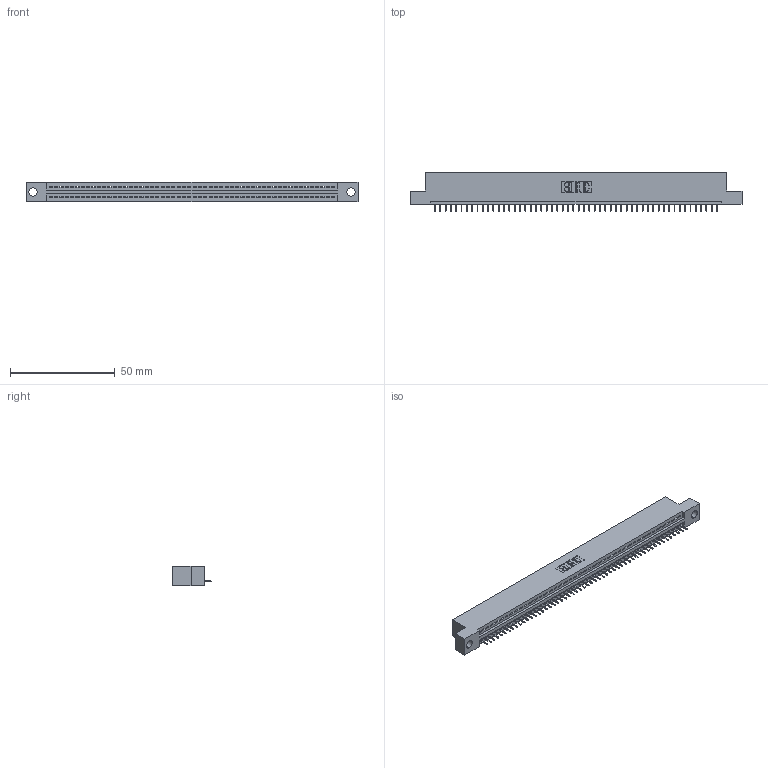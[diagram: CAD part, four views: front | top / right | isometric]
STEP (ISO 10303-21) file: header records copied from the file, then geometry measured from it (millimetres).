
FILE_DESCRIPTION (( 'STEP AP203' ), '1' );
FILE_NAME ('895-054-525-104.STEP', '2020-09-27T13:54:19', ( '' ), ( '' ), 'SwSTEP 2.0', 'SolidWorks 2020', '' );
FILE_SCHEMA (( 'CONFIG_CONTROL_DESIGN' ));
Length unit declared in the file: inch
Products named in the file (3): 345-292-001_345-293-125; 845 Part_Flush Mounting Lugs - 0.156 Dia-TH; 895-054-525-104
Assembly tree (55 placements, depth 2):
  895-054-525-104
    845 Part_Flush Mounting Lugs - 0.156 Dia-TH
    345-292-001_345-293-125  x54
Bounding box: 158.37 x 18.72 x 9.4 mm (x, y, z)
Volume: 14832 mm3; surface area: 18947 mm2
Topology: 55 solids, 55 shells, 3474 faces, 10061 edges, 6490 vertices
Faces by surface type: plane 2564, cylinder 910
Entity records: 39103 total; most frequent: CARTESIAN_POINT 6778, ORIENTED_EDGE 6766, DIRECTION 5903, EDGE_CURVE 3383, VECTOR 3039, LINE 3039, VERTEX_POINT 2250, AXIS2_PLACEMENT_3D 1432
